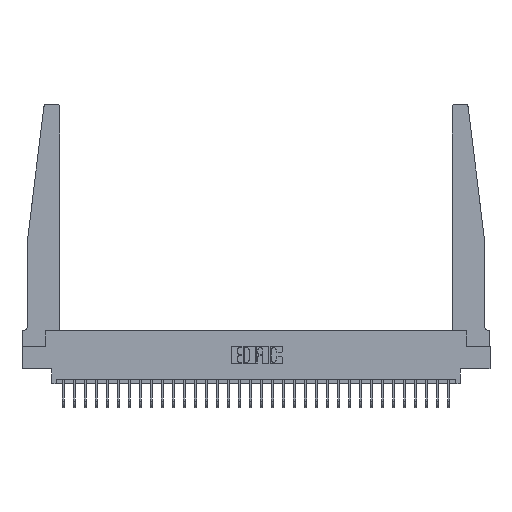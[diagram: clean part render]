
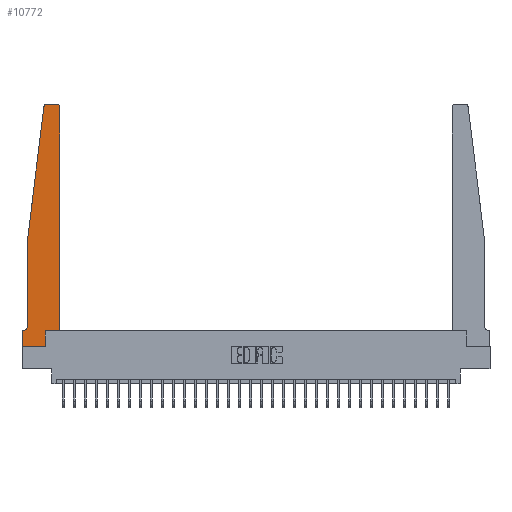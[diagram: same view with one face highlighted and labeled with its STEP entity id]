
A CAD part, top view. The second image highlights one B-rep face of the part: STEP entity #10772.
In plain terms, the highlighted planar face has unit normal (0, 0, 1).
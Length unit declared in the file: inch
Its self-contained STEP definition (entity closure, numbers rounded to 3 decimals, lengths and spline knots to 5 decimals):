
#97 = VERTEX_POINT ( 'NONE', #9938 ) ;
#603 = CARTESIAN_POINT ( 'NONE',  ( 0.015, 0.2375, 0.37 ) ) ;
#665 = CARTESIAN_POINT ( 'NONE',  ( 0.24675, 2.72367, 0.37 ) ) ;
#803 = CARTESIAN_POINT ( 'NONE',  ( 0.065, 1.25, 0.37 ) ) ;
#1035 = ORIENTED_EDGE ( 'NONE', *, *, #15105, .T. ) ;
#1046 = CIRCLE ( 'NONE', #23861, 0.03 ) ;
#1192 = CARTESIAN_POINT ( 'NONE',  ( 0.065, 0.1875, 0.37 ) ) ;
#1547 = CARTESIAN_POINT ( 'NONE',  ( 0., 0.1875, 0.37 ) ) ;
#1571 = ORIENTED_EDGE ( 'NONE', *, *, #15792, .T. ) ;
#1625 = ORIENTED_EDGE ( 'NONE', *, *, #17687, .T. ) ;
#1955 = VERTEX_POINT ( 'NONE', #23348 ) ;
#2017 = ORIENTED_EDGE ( 'NONE', *, *, #21884, .T. ) ;
#2369 = VERTEX_POINT ( 'NONE', #9649 ) ;
#2694 = ORIENTED_EDGE ( 'NONE', *, *, #6125, .T. ) ;
#2854 = DIRECTION ( 'NONE',  ( -1., 0., 0. ) ) ;
#3794 = ORIENTED_EDGE ( 'NONE', *, *, #25743, .T. ) ;
#3804 = PLANE ( 'NONE',  #17777 ) ;
#3859 = ORIENTED_EDGE ( 'NONE', *, *, #23434, .T. ) ;
#3922 = ORIENTED_EDGE ( 'NONE', *, *, #19385, .T. ) ;
#4498 = CARTESIAN_POINT ( 'NONE',  ( 0., 0.1875, 0.37 ) ) ;
#4610 = ORIENTED_EDGE ( 'NONE', *, *, #12480, .T. ) ;
#4727 = CARTESIAN_POINT ( 'NONE',  ( 0.25, 2.75, 0.37 ) ) ;
#4964 = ORIENTED_EDGE ( 'NONE', *, *, #13771, .T. ) ;
#5056 = CARTESIAN_POINT ( 'NONE',  ( 0.27653, 2.72, 0.37 ) ) ;
#5343 = DIRECTION ( 'NONE',  ( 1., 0., 0. ) ) ;
#5840 = VECTOR ( 'NONE', #26173, 39.37008 ) ;
#6014 = DIRECTION ( 'NONE',  ( 0., 0., 1. ) ) ;
#6125 = EDGE_CURVE ( 'NONE', #2369, #13217, #1046, .T. ) ;
#6350 = LINE ( 'NONE', #1192, #27986 ) ;
#7231 = DIRECTION ( 'NONE',  ( 1., 0., 0. ) ) ;
#7276 = LINE ( 'NONE', #20596, #18116 ) ;
#7388 = ORIENTED_EDGE ( 'NONE', *, *, #15701, .T. ) ;
#8064 = ORIENTED_EDGE ( 'NONE', *, *, #8066, .T. ) ;
#8066 = EDGE_CURVE ( 'NONE', #19485, #18709, #10606, .T. ) ;
#8305 = CARTESIAN_POINT ( 'NONE',  ( 0.2605, 0.18, 0.37 ) ) ;
#8581 = VERTEX_POINT ( 'NONE', #15726 ) ;
#8900 = CARTESIAN_POINT ( 'NONE',  ( 0.425, 0.18, 0.37 ) ) ;
#8976 = CARTESIAN_POINT ( 'NONE',  ( 0.395, 2.72, 0.37 ) ) ;
#9209 = AXIS2_PLACEMENT_3D ( 'NONE', #8976, #24068, #11158 ) ;
#9649 = CARTESIAN_POINT ( 'NONE',  ( 0.27653, 2.75, 0.37 ) ) ;
#9877 = VECTOR ( 'NONE', #24212, 39.37008 ) ;
#9938 = CARTESIAN_POINT ( 'NONE',  ( 0.425, 2.72, 0.37 ) ) ;
#10008 = FACE_OUTER_BOUND ( 'NONE', #24761, .T. ) ;
#10606 = LINE ( 'NONE', #16139, #27136 ) ;
#10772 = ADVANCED_FACE ( 'NONE', ( #10008 ), #3804, .T. ) ;
#10937 = CARTESIAN_POINT ( 'NONE',  ( 0.2605, 0., 0.37 ) ) ;
#11158 = DIRECTION ( 'NONE',  ( 1., 0., 0. ) ) ;
#11303 = CARTESIAN_POINT ( 'NONE',  ( 0.065, 1.25, 0.37 ) ) ;
#11445 = LINE ( 'NONE', #803, #16531 ) ;
#11454 = CARTESIAN_POINT ( 'NONE',  ( 0., 0., 0.37 ) ) ;
#11839 = LINE ( 'NONE', #13478, #21977 ) ;
#12480 = EDGE_CURVE ( 'NONE', #1955, #8581, #23789, .T. ) ;
#12801 = LINE ( 'NONE', #13635, #23615 ) ;
#13217 = VERTEX_POINT ( 'NONE', #665 ) ;
#13290 = CARTESIAN_POINT ( 'NONE',  ( 0.425, 0.18, 0.37 ) ) ;
#13478 = CARTESIAN_POINT ( 'NONE',  ( 0.425, 0.18, 0.37 ) ) ;
#13635 = CARTESIAN_POINT ( 'NONE',  ( 0.065, 1.25, 0.37 ) ) ;
#13771 = EDGE_CURVE ( 'NONE', #18350, #2369, #15619, .T. ) ;
#15105 = EDGE_CURVE ( 'NONE', #26899, #97, #11839, .T. ) ;
#15457 = DIRECTION ( 'NONE',  ( 0., 1., 0. ) ) ;
#15619 = LINE ( 'NONE', #4727, #9877 ) ;
#15701 = EDGE_CURVE ( 'NONE', #20663, #1955, #12801, .T. ) ;
#15726 = CARTESIAN_POINT ( 'NONE',  ( 0.015, 0.1875, 0.37 ) ) ;
#15792 = EDGE_CURVE ( 'NONE', #13217, #20663, #11445, .T. ) ;
#15888 = DIRECTION ( 'NONE',  ( 0., 0., -1. ) ) ;
#16084 = DIRECTION ( 'NONE',  ( -0.122, -0.992, 0. ) ) ;
#16139 = CARTESIAN_POINT ( 'NONE',  ( 0., 0., 0.37 ) ) ;
#16461 = DIRECTION ( 'NONE',  ( -1., 0., 0. ) ) ;
#16531 = VECTOR ( 'NONE', #16084, 39.37008 ) ;
#17687 = EDGE_CURVE ( 'NONE', #22215, #26899, #18135, .T. ) ;
#17777 = AXIS2_PLACEMENT_3D ( 'NONE', #1547, #6014, #21160 ) ;
#18116 = VECTOR ( 'NONE', #26989, 39.37008 ) ;
#18135 = LINE ( 'NONE', #8900, #23867 ) ;
#18350 = VERTEX_POINT ( 'NONE', #24721 ) ;
#18709 = VERTEX_POINT ( 'NONE', #10937 ) ;
#19385 = EDGE_CURVE ( 'NONE', #18709, #22215, #23103, .T. ) ;
#19485 = VERTEX_POINT ( 'NONE', #11454 ) ;
#20200 = DIRECTION ( 'NONE',  ( 0., 0., 1. ) ) ;
#20596 = CARTESIAN_POINT ( 'NONE',  ( 0., 0., 0.37 ) ) ;
#20663 = VERTEX_POINT ( 'NONE', #11303 ) ;
#21160 = DIRECTION ( 'NONE',  ( 1., 0., 0. ) ) ;
#21865 = CARTESIAN_POINT ( 'NONE',  ( 0.2605, 0.18, 0.37 ) ) ;
#21884 = EDGE_CURVE ( 'NONE', #97, #18350, #22319, .T. ) ;
#21977 = VECTOR ( 'NONE', #15457, 39.37008 ) ;
#22215 = VERTEX_POINT ( 'NONE', #8305 ) ;
#22319 = CIRCLE ( 'NONE', #9209, 0.03 ) ;
#22343 = AXIS2_PLACEMENT_3D ( 'NONE', #603, #15888, #2854 ) ;
#23103 = LINE ( 'NONE', #21865, #5840 ) ;
#23348 = CARTESIAN_POINT ( 'NONE',  ( 0.065, 0.2375, 0.37 ) ) ;
#23434 = EDGE_CURVE ( 'NONE', #8581, #27434, #6350, .T. ) ;
#23615 = VECTOR ( 'NONE', #26538, 39.37008 ) ;
#23789 = CIRCLE ( 'NONE', #22343, 0.05 ) ;
#23861 = AXIS2_PLACEMENT_3D ( 'NONE', #5056, #20200, #7231 ) ;
#23867 = VECTOR ( 'NONE', #23998, 39.37008 ) ;
#23998 = DIRECTION ( 'NONE',  ( 1., 0., 0. ) ) ;
#24068 = DIRECTION ( 'NONE',  ( 0., 0., 1. ) ) ;
#24212 = DIRECTION ( 'NONE',  ( -1., 0., 0. ) ) ;
#24721 = CARTESIAN_POINT ( 'NONE',  ( 0.395, 2.75, 0.37 ) ) ;
#24761 = EDGE_LOOP ( 'NONE', ( #4964, #2694, #1571, #7388, #4610, #3859, #3794, #8064, #3922, #1625, #1035, #2017 ) ) ;
#25743 = EDGE_CURVE ( 'NONE', #27434, #19485, #7276, .T. ) ;
#26173 = DIRECTION ( 'NONE',  ( 0., 1., 0. ) ) ;
#26538 = DIRECTION ( 'NONE',  ( 0., -1., 0. ) ) ;
#26899 = VERTEX_POINT ( 'NONE', #13290 ) ;
#26989 = DIRECTION ( 'NONE',  ( 0., -1., 0. ) ) ;
#27136 = VECTOR ( 'NONE', #5343, 39.37008 ) ;
#27434 = VERTEX_POINT ( 'NONE', #4498 ) ;
#27986 = VECTOR ( 'NONE', #16461, 39.37008 ) ;
